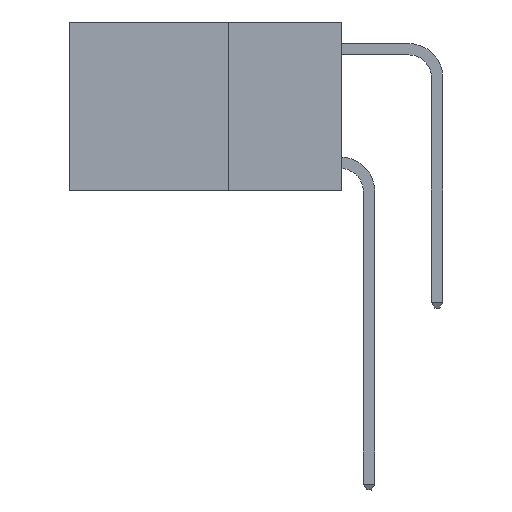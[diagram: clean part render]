
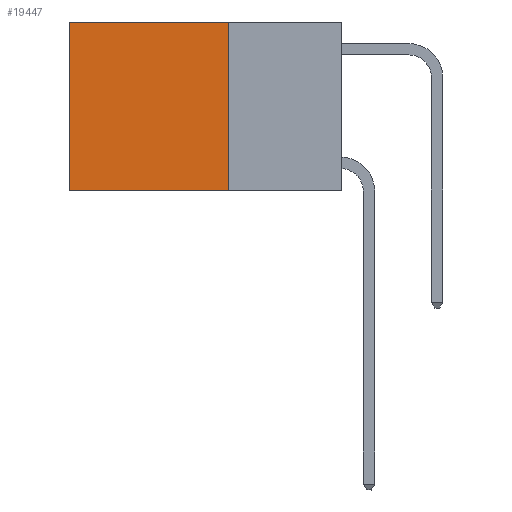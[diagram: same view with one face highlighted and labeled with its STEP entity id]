
A CAD part, left-side view. The second image highlights one B-rep face of the part: STEP entity #19447.
In plain terms, the highlighted planar face has unit normal (-1, 0, 0).
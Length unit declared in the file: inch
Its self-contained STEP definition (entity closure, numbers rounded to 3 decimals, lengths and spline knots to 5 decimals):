
#1093 = EDGE_CURVE ( 'NONE', #1351, #10643, #19515, .T. ) ;
#1150 = DIRECTION ( 'NONE',  ( 0., 0., -1. ) ) ;
#1351 = VERTEX_POINT ( 'NONE', #16379 ) ;
#2021 = ORIENTED_EDGE ( 'NONE', *, *, #20406, .F. ) ;
#2139 = VERTEX_POINT ( 'NONE', #19892 ) ;
#2153 = VECTOR ( 'NONE', #10393, 39.37008 ) ;
#5127 = FACE_OUTER_BOUND ( 'NONE', #7002, .T. ) ;
#5429 = CARTESIAN_POINT ( 'NONE',  ( 0.2625, 0.6, 0. ) ) ;
#5748 = ORIENTED_EDGE ( 'NONE', *, *, #8097, .T. ) ;
#6263 = PLANE ( 'NONE',  #14485 ) ;
#7002 = EDGE_LOOP ( 'NONE', ( #5748, #2021, #18716, #16377 ) ) ;
#7275 = CARTESIAN_POINT ( 'NONE',  ( 0.2625, 0.25, -0.37 ) ) ;
#7406 = VECTOR ( 'NONE', #1150, 39.37008 ) ;
#8097 = EDGE_CURVE ( 'NONE', #10643, #11306, #20944, .T. ) ;
#9666 = DIRECTION ( 'NONE',  ( 0., 0., -1. ) ) ;
#9803 = CARTESIAN_POINT ( 'NONE',  ( 0.2625, 0.25, 0. ) ) ;
#10346 = DIRECTION ( 'NONE',  ( 0., 0., -1. ) ) ;
#10393 = DIRECTION ( 'NONE',  ( 0., 1., 0. ) ) ;
#10505 = CARTESIAN_POINT ( 'NONE',  ( 0.2625, 0.6, -0.37 ) ) ;
#10643 = VERTEX_POINT ( 'NONE', #5429 ) ;
#11306 = VERTEX_POINT ( 'NONE', #10505 ) ;
#12637 = CARTESIAN_POINT ( 'NONE',  ( 0.2625, 0.6, 0. ) ) ;
#13270 = LINE ( 'NONE', #7275, #2153 ) ;
#13432 = EDGE_CURVE ( 'NONE', #1351, #2139, #16173, .T. ) ;
#13599 = DIRECTION ( 'NONE',  ( 1., 0., 0. ) ) ;
#14485 = AXIS2_PLACEMENT_3D ( 'NONE', #18662, #13599, #10346 ) ;
#16173 = LINE ( 'NONE', #17991, #17761 ) ;
#16377 = ORIENTED_EDGE ( 'NONE', *, *, #1093, .T. ) ;
#16379 = CARTESIAN_POINT ( 'NONE',  ( 0.2625, 0.25, 0. ) ) ;
#16858 = DIRECTION ( 'NONE',  ( 0., 1., 0. ) ) ;
#17761 = VECTOR ( 'NONE', #9666, 39.37008 ) ;
#17991 = CARTESIAN_POINT ( 'NONE',  ( 0.2625, 0.25, 0. ) ) ;
#18662 = CARTESIAN_POINT ( 'NONE',  ( 0.2625, 0.25, 0. ) ) ;
#18716 = ORIENTED_EDGE ( 'NONE', *, *, #13432, .F. ) ;
#19447 = ADVANCED_FACE ( 'NONE', ( #5127 ), #6263, .F. ) ;
#19515 = LINE ( 'NONE', #9803, #21113 ) ;
#19892 = CARTESIAN_POINT ( 'NONE',  ( 0.2625, 0.25, -0.37 ) ) ;
#20406 = EDGE_CURVE ( 'NONE', #2139, #11306, #13270, .T. ) ;
#20944 = LINE ( 'NONE', #12637, #7406 ) ;
#21113 = VECTOR ( 'NONE', #16858, 39.37008 ) ;
